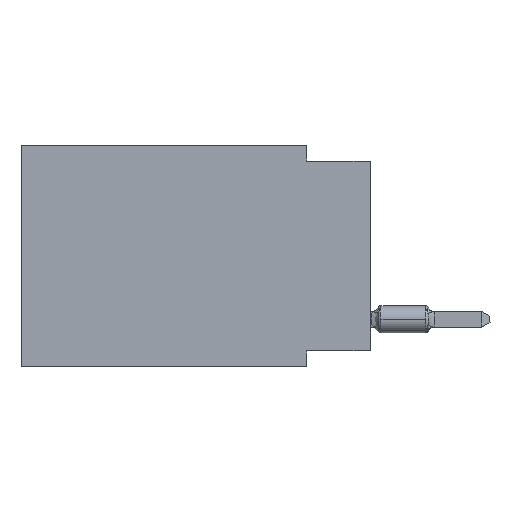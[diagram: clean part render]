
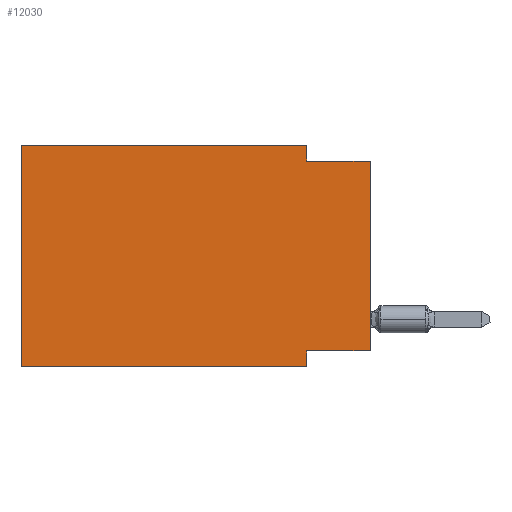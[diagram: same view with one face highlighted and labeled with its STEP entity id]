
A CAD part, left-side view. The second image highlights one B-rep face of the part: STEP entity #12030.
In plain terms, the highlighted planar face has unit normal (-1, 0, 0).
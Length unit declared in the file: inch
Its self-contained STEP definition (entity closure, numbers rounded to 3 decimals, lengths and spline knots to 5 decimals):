
#139 = ORIENTED_EDGE ( 'NONE', *, *, #9044, .T. ) ;
#190 = LINE ( 'NONE', #996, #12654 ) ;
#204 = LINE ( 'NONE', #9730, #7823 ) ;
#834 = EDGE_CURVE ( 'NONE', #8267, #7945, #2276, .T. ) ;
#996 = CARTESIAN_POINT ( 'NONE',  ( 0., 0.55, -0.35 ) ) ;
#1123 = VECTOR ( 'NONE', #8461, 39.37008 ) ;
#1439 = CARTESIAN_POINT ( 'NONE',  ( 0., 0., -0.025 ) ) ;
#2121 = CARTESIAN_POINT ( 'NONE',  ( 0., 0.55, 0. ) ) ;
#2276 = LINE ( 'NONE', #1439, #10434 ) ;
#3224 = LINE ( 'NONE', #2121, #7353 ) ;
#3252 = ORIENTED_EDGE ( 'NONE', *, *, #9517, .F. ) ;
#3990 = VERTEX_POINT ( 'NONE', #5234 ) ;
#4466 = DIRECTION ( 'NONE',  ( 0., -1., 0. ) ) ;
#4507 = LINE ( 'NONE', #6268, #1123 ) ;
#4611 = CARTESIAN_POINT ( 'NONE',  ( 0., 0., -0.025 ) ) ;
#5234 = CARTESIAN_POINT ( 'NONE',  ( 0., 0., -0.325 ) ) ;
#5373 = EDGE_LOOP ( 'NONE', ( #10192, #11648, #5532, #13247, #5421, #139, #8199, #3252 ) ) ;
#5421 = ORIENTED_EDGE ( 'NONE', *, *, #8112, .F. ) ;
#5532 = ORIENTED_EDGE ( 'NONE', *, *, #13550, .F. ) ;
#5628 = CARTESIAN_POINT ( 'NONE',  ( 0., 0.1, 0. ) ) ;
#6108 = EDGE_CURVE ( 'NONE', #10460, #6339, #3224, .T. ) ;
#6268 = CARTESIAN_POINT ( 'NONE',  ( 0., 0., 0. ) ) ;
#6337 = CARTESIAN_POINT ( 'NONE',  ( 0., 0.1, -0.025 ) ) ;
#6339 = VERTEX_POINT ( 'NONE', #5628 ) ;
#6640 = LINE ( 'NONE', #10115, #10988 ) ;
#6845 = PLANE ( 'NONE',  #7289 ) ;
#6967 = DIRECTION ( 'NONE',  ( 0., 1., 0. ) ) ;
#6975 = CARTESIAN_POINT ( 'NONE',  ( 0., 0.55, 0. ) ) ;
#7289 = AXIS2_PLACEMENT_3D ( 'NONE', #6975, #12200, #8993 ) ;
#7353 = VECTOR ( 'NONE', #10577, 39.37008 ) ;
#7563 = CARTESIAN_POINT ( 'NONE',  ( 0., 0.1, 0. ) ) ;
#7636 = VECTOR ( 'NONE', #12448, 39.37008 ) ;
#7715 = EDGE_CURVE ( 'NONE', #3990, #7945, #4507, .T. ) ;
#7823 = VECTOR ( 'NONE', #8740, 39.37008 ) ;
#7945 = VERTEX_POINT ( 'NONE', #4611 ) ;
#8026 = VERTEX_POINT ( 'NONE', #11262 ) ;
#8112 = EDGE_CURVE ( 'NONE', #8026, #10460, #11148, .T. ) ;
#8199 = ORIENTED_EDGE ( 'NONE', *, *, #8660, .F. ) ;
#8221 = LINE ( 'NONE', #7563, #9728 ) ;
#8267 = VERTEX_POINT ( 'NONE', #6337 ) ;
#8399 = VERTEX_POINT ( 'NONE', #11172 ) ;
#8461 = DIRECTION ( 'NONE',  ( 0., 0., 1. ) ) ;
#8538 = CARTESIAN_POINT ( 'NONE',  ( 0., 0.1, -0.35 ) ) ;
#8660 = EDGE_CURVE ( 'NONE', #8399, #9208, #204, .T. ) ;
#8740 = DIRECTION ( 'NONE',  ( 0., 0., -1. ) ) ;
#8993 = DIRECTION ( 'NONE',  ( 0., 0., -1. ) ) ;
#9044 = EDGE_CURVE ( 'NONE', #8026, #9208, #190, .T. ) ;
#9208 = VERTEX_POINT ( 'NONE', #8538 ) ;
#9339 = DIRECTION ( 'NONE',  ( 0., -1., 0. ) ) ;
#9517 = EDGE_CURVE ( 'NONE', #3990, #8399, #6640, .T. ) ;
#9728 = VECTOR ( 'NONE', #12954, 39.37008 ) ;
#9730 = CARTESIAN_POINT ( 'NONE',  ( 0., 0.1, -0.35 ) ) ;
#10115 = CARTESIAN_POINT ( 'NONE',  ( 0., 0., -0.325 ) ) ;
#10192 = ORIENTED_EDGE ( 'NONE', *, *, #7715, .T. ) ;
#10434 = VECTOR ( 'NONE', #4466, 39.37008 ) ;
#10460 = VERTEX_POINT ( 'NONE', #12209 ) ;
#10515 = CARTESIAN_POINT ( 'NONE',  ( 0., 0.55, 0. ) ) ;
#10577 = DIRECTION ( 'NONE',  ( 0., -1., 0. ) ) ;
#10988 = VECTOR ( 'NONE', #6967, 39.37008 ) ;
#11148 = LINE ( 'NONE', #10515, #7636 ) ;
#11172 = CARTESIAN_POINT ( 'NONE',  ( 0., 0.1, -0.325 ) ) ;
#11262 = CARTESIAN_POINT ( 'NONE',  ( 0., 0.55, -0.35 ) ) ;
#11648 = ORIENTED_EDGE ( 'NONE', *, *, #834, .F. ) ;
#12030 = ADVANCED_FACE ( 'NONE', ( #13403 ), #6845, .F. ) ;
#12200 = DIRECTION ( 'NONE',  ( 1., 0., 0. ) ) ;
#12209 = CARTESIAN_POINT ( 'NONE',  ( 0., 0.55, 0. ) ) ;
#12448 = DIRECTION ( 'NONE',  ( 0., 0., 1. ) ) ;
#12654 = VECTOR ( 'NONE', #9339, 39.37008 ) ;
#12954 = DIRECTION ( 'NONE',  ( 0., 0., -1. ) ) ;
#13247 = ORIENTED_EDGE ( 'NONE', *, *, #6108, .F. ) ;
#13403 = FACE_OUTER_BOUND ( 'NONE', #5373, .T. ) ;
#13550 = EDGE_CURVE ( 'NONE', #6339, #8267, #8221, .T. ) ;
